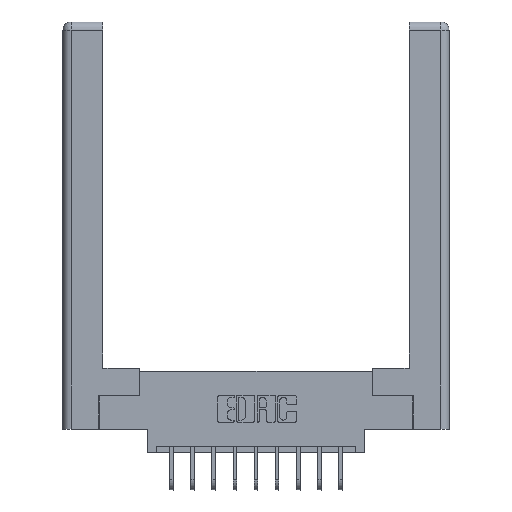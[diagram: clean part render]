
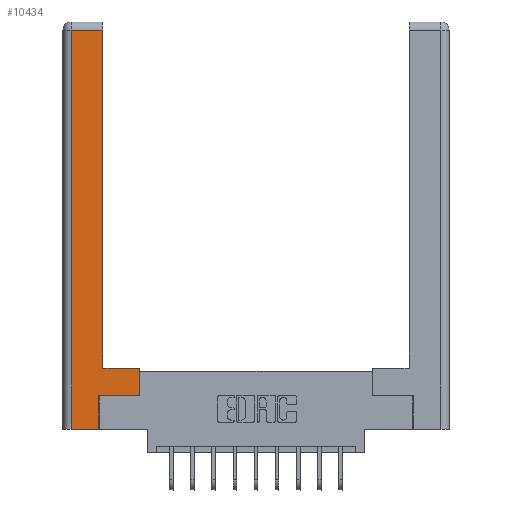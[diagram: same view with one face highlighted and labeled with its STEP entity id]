
A CAD part, top view. The second image highlights one B-rep face of the part: STEP entity #10434.
In plain terms, the highlighted planar face has unit normal (0, 0, 1).
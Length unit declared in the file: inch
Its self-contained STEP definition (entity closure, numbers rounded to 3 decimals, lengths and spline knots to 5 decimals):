
#797 = EDGE_CURVE ( 'NONE', #4678, #5167, #2208, .T. ) ;
#809 = ORIENTED_EDGE ( 'NONE', *, *, #13234, .T. ) ;
#812 = CARTESIAN_POINT ( 'NONE',  ( 0.295, 0.45, 0. ) ) ;
#1281 = DIRECTION ( 'NONE',  ( 1., 0., 0. ) ) ;
#1408 = VERTEX_POINT ( 'NONE', #1458 ) ;
#1410 = CARTESIAN_POINT ( 'NONE',  ( 0.295, 3., 0. ) ) ;
#1458 = CARTESIAN_POINT ( 'NONE',  ( 0.295, 0.45, 0. ) ) ;
#1755 = DIRECTION ( 'NONE',  ( 0., -1., 0. ) ) ;
#1759 = LINE ( 'NONE', #7568, #12081 ) ;
#2208 = LINE ( 'NONE', #9902, #12195 ) ;
#2363 = LINE ( 'NONE', #13383, #7216 ) ;
#2366 = FACE_OUTER_BOUND ( 'NONE', #3288, .T. ) ;
#2435 = ORIENTED_EDGE ( 'NONE', *, *, #9835, .T. ) ;
#2442 = DIRECTION ( 'NONE',  ( 0., 1., 0. ) ) ;
#2481 = DIRECTION ( 'NONE',  ( 0., 1., 0. ) ) ;
#2636 = VECTOR ( 'NONE', #2481, 39.37008 ) ;
#3009 = CARTESIAN_POINT ( 'NONE',  ( 0.565, 0.45, 0. ) ) ;
#3288 = EDGE_LOOP ( 'NONE', ( #13729, #7364, #2435, #13233, #10173, #13368, #809, #5934 ) ) ;
#4278 = VERTEX_POINT ( 'NONE', #6774 ) ;
#4330 = CARTESIAN_POINT ( 'NONE',  ( 0.565, 0.245, 0. ) ) ;
#4571 = VECTOR ( 'NONE', #8289, 39.37008 ) ;
#4678 = VERTEX_POINT ( 'NONE', #10422 ) ;
#4718 = EDGE_CURVE ( 'NONE', #11561, #4678, #1759, .T. ) ;
#5109 = DIRECTION ( 'NONE',  ( -1., 0., 0. ) ) ;
#5167 = VERTEX_POINT ( 'NONE', #10011 ) ;
#5890 = LINE ( 'NONE', #3009, #9729 ) ;
#5934 = ORIENTED_EDGE ( 'NONE', *, *, #9376, .T. ) ;
#6326 = EDGE_CURVE ( 'NONE', #5167, #4278, #8317, .T. ) ;
#6494 = DIRECTION ( 'NONE',  ( 1., 0., 0. ) ) ;
#6499 = EDGE_CURVE ( 'NONE', #1408, #12854, #11114, .T. ) ;
#6555 = VERTEX_POINT ( 'NONE', #12071 ) ;
#6774 = CARTESIAN_POINT ( 'NONE',  ( 0.565, 0.245, 0. ) ) ;
#6872 = VECTOR ( 'NONE', #5109, 39.37008 ) ;
#7003 = DIRECTION ( 'NONE',  ( -1., 0., 0. ) ) ;
#7103 = CARTESIAN_POINT ( 'NONE',  ( 0., 0., 0. ) ) ;
#7216 = VECTOR ( 'NONE', #1755, 39.37008 ) ;
#7364 = ORIENTED_EDGE ( 'NONE', *, *, #9853, .T. ) ;
#7467 = CARTESIAN_POINT ( 'NONE',  ( 0.0615, 2.94, 0. ) ) ;
#7568 = CARTESIAN_POINT ( 'NONE',  ( 0.265, 0., 0. ) ) ;
#8289 = DIRECTION ( 'NONE',  ( -1., 0., 0. ) ) ;
#8317 = LINE ( 'NONE', #4330, #13640 ) ;
#9232 = LINE ( 'NONE', #812, #4571 ) ;
#9376 = EDGE_CURVE ( 'NONE', #6555, #1408, #9232, .T. ) ;
#9399 = CARTESIAN_POINT ( 'NONE',  ( 0.0615, 2.94, 0. ) ) ;
#9729 = VECTOR ( 'NONE', #10473, 39.37008 ) ;
#9835 = EDGE_CURVE ( 'NONE', #10689, #11561, #2363, .T. ) ;
#9853 = EDGE_CURVE ( 'NONE', #12854, #10689, #11517, .T. ) ;
#9902 = CARTESIAN_POINT ( 'NONE',  ( 0.265, 0.245, 0. ) ) ;
#10011 = CARTESIAN_POINT ( 'NONE',  ( 0.265, 0.245, 0. ) ) ;
#10173 = ORIENTED_EDGE ( 'NONE', *, *, #797, .T. ) ;
#10193 = DIRECTION ( 'NONE',  ( 0., 0., -1. ) ) ;
#10422 = CARTESIAN_POINT ( 'NONE',  ( 0.265, 0., 0. ) ) ;
#10434 = ADVANCED_FACE ( 'NONE', ( #2366 ), #12442, .F. ) ;
#10473 = DIRECTION ( 'NONE',  ( 0., 1., 0. ) ) ;
#10689 = VERTEX_POINT ( 'NONE', #7467 ) ;
#11114 = LINE ( 'NONE', #1410, #2636 ) ;
#11517 = LINE ( 'NONE', #9399, #6872 ) ;
#11561 = VERTEX_POINT ( 'NONE', #13656 ) ;
#11950 = CARTESIAN_POINT ( 'NONE',  ( 0.295, 2.94, 0. ) ) ;
#12071 = CARTESIAN_POINT ( 'NONE',  ( 0.565, 0.45, 0. ) ) ;
#12081 = VECTOR ( 'NONE', #1281, 39.37008 ) ;
#12195 = VECTOR ( 'NONE', #2442, 39.37008 ) ;
#12291 = AXIS2_PLACEMENT_3D ( 'NONE', #7103, #10193, #7003 ) ;
#12442 = PLANE ( 'NONE',  #12291 ) ;
#12854 = VERTEX_POINT ( 'NONE', #11950 ) ;
#13233 = ORIENTED_EDGE ( 'NONE', *, *, #4718, .T. ) ;
#13234 = EDGE_CURVE ( 'NONE', #4278, #6555, #5890, .T. ) ;
#13368 = ORIENTED_EDGE ( 'NONE', *, *, #6326, .T. ) ;
#13383 = CARTESIAN_POINT ( 'NONE',  ( 0.0615, 0., 0. ) ) ;
#13640 = VECTOR ( 'NONE', #6494, 39.37008 ) ;
#13656 = CARTESIAN_POINT ( 'NONE',  ( 0.0615, 0., 0. ) ) ;
#13729 = ORIENTED_EDGE ( 'NONE', *, *, #6499, .T. ) ;
